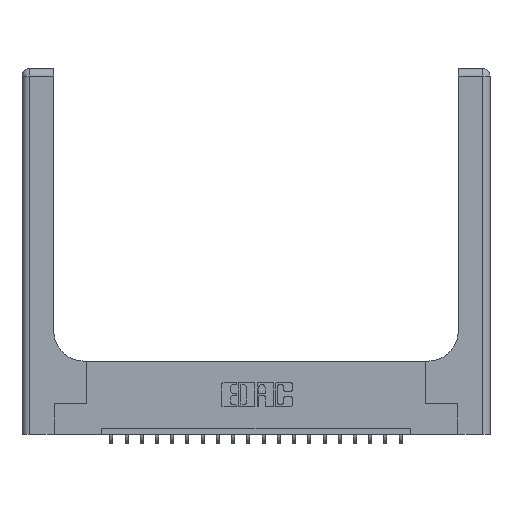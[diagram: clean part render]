
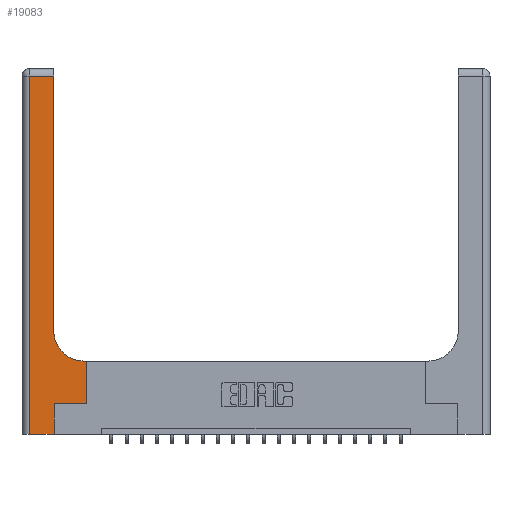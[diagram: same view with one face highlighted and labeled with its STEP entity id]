
A CAD part, top view. The second image highlights one B-rep face of the part: STEP entity #19083.
In plain terms, the highlighted planar face has unit normal (0, 0, 1).
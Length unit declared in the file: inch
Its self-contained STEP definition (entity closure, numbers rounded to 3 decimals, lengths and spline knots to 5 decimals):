
#293 = DIRECTION ( 'NONE',  ( 1., 0., 0. ) ) ;
#613 = DIRECTION ( 'NONE',  ( 0., 0., -1. ) ) ;
#1088 = VECTOR ( 'NONE', #14825, 39.37008 ) ;
#1104 = CARTESIAN_POINT ( 'NONE',  ( 0., 2.94, 0.37 ) ) ;
#1169 = ORIENTED_EDGE ( 'NONE', *, *, #7126, .T. ) ;
#1303 = VECTOR ( 'NONE', #6247, 39.37008 ) ;
#1861 = VERTEX_POINT ( 'NONE', #7684 ) ;
#1907 = CARTESIAN_POINT ( 'NONE',  ( 0.51, 0.85, 0.37 ) ) ;
#2509 = DIRECTION ( 'NONE',  ( -1., 0., 0. ) ) ;
#2930 = ORIENTED_EDGE ( 'NONE', *, *, #20727, .T. ) ;
#3854 = ORIENTED_EDGE ( 'NONE', *, *, #9664, .T. ) ;
#4037 = EDGE_CURVE ( 'NONE', #7189, #21075, #8366, .T. ) ;
#4624 = FACE_OUTER_BOUND ( 'NONE', #9613, .T. ) ;
#4665 = EDGE_CURVE ( 'NONE', #15276, #17112, #15567, .T. ) ;
#4895 = VERTEX_POINT ( 'NONE', #20072 ) ;
#6247 = DIRECTION ( 'NONE',  ( 0., -1., 0. ) ) ;
#6310 = CARTESIAN_POINT ( 'NONE',  ( 0.26, 3., 0.37 ) ) ;
#6574 = CARTESIAN_POINT ( 'NONE',  ( 0.26, 0.6, 0.37 ) ) ;
#6630 = CARTESIAN_POINT ( 'NONE',  ( 0.528, 0.25, 0.37 ) ) ;
#6782 = LINE ( 'NONE', #6574, #1088 ) ;
#7012 = ORIENTED_EDGE ( 'NONE', *, *, #15500, .T. ) ;
#7126 = EDGE_CURVE ( 'NONE', #17112, #9263, #20725, .T. ) ;
#7189 = VERTEX_POINT ( 'NONE', #19460 ) ;
#7630 = PLANE ( 'NONE',  #12415 ) ;
#7684 = CARTESIAN_POINT ( 'NONE',  ( 0.26, 0.85, 0.37 ) ) ;
#7922 = VECTOR ( 'NONE', #16930, 39.37008 ) ;
#7959 = VERTEX_POINT ( 'NONE', #14280 ) ;
#8366 = LINE ( 'NONE', #18451, #14197 ) ;
#8649 = CARTESIAN_POINT ( 'NONE',  ( 0.265, 0., 0.37 ) ) ;
#8744 = ORIENTED_EDGE ( 'NONE', *, *, #4037, .T. ) ;
#8818 = EDGE_CURVE ( 'NONE', #21075, #4895, #17923, .T. ) ;
#9263 = VERTEX_POINT ( 'NONE', #14306 ) ;
#9374 = EDGE_CURVE ( 'NONE', #7959, #1861, #20838, .T. ) ;
#9612 = CARTESIAN_POINT ( 'NONE',  ( 0.06, 2.94, 0.37 ) ) ;
#9613 = EDGE_LOOP ( 'NONE', ( #2930, #11601, #1169, #10731, #7012, #8744, #12148, #3854, #19060 ) ) ;
#9664 = EDGE_CURVE ( 'NONE', #4895, #7959, #6782, .T. ) ;
#10173 = DIRECTION ( 'NONE',  ( 1., 0., 0. ) ) ;
#10459 = LINE ( 'NONE', #8649, #7922 ) ;
#10731 = ORIENTED_EDGE ( 'NONE', *, *, #20761, .T. ) ;
#11212 = CARTESIAN_POINT ( 'NONE',  ( 0.528, 0.25, 0.37 ) ) ;
#11262 = CARTESIAN_POINT ( 'NONE',  ( 0., 3., 0.37 ) ) ;
#11339 = AXIS2_PLACEMENT_3D ( 'NONE', #1907, #613, #293 ) ;
#11601 = ORIENTED_EDGE ( 'NONE', *, *, #4665, .T. ) ;
#11737 = VECTOR ( 'NONE', #12838, 39.37008 ) ;
#12148 = ORIENTED_EDGE ( 'NONE', *, *, #8818, .T. ) ;
#12415 = AXIS2_PLACEMENT_3D ( 'NONE', #11262, #20925, #14150 ) ;
#12625 = LINE ( 'NONE', #6310, #11737 ) ;
#12838 = DIRECTION ( 'NONE',  ( 0., 1., 0. ) ) ;
#13162 = DIRECTION ( 'NONE',  ( 0., 1., 0. ) ) ;
#14006 = VECTOR ( 'NONE', #13162, 39.37008 ) ;
#14150 = DIRECTION ( 'NONE',  ( -1., 0., 0. ) ) ;
#14197 = VECTOR ( 'NONE', #10173, 39.37008 ) ;
#14280 = CARTESIAN_POINT ( 'NONE',  ( 0.51, 0.6, 0.37 ) ) ;
#14306 = CARTESIAN_POINT ( 'NONE',  ( 0.06, 0., 0.37 ) ) ;
#14825 = DIRECTION ( 'NONE',  ( -1., 0., 0. ) ) ;
#15276 = VERTEX_POINT ( 'NONE', #17991 ) ;
#15500 = EDGE_CURVE ( 'NONE', #15914, #7189, #10459, .T. ) ;
#15567 = LINE ( 'NONE', #1104, #18614 ) ;
#15914 = VERTEX_POINT ( 'NONE', #18074 ) ;
#16930 = DIRECTION ( 'NONE',  ( 0., 1., 0. ) ) ;
#17112 = VERTEX_POINT ( 'NONE', #9612 ) ;
#17923 = LINE ( 'NONE', #6630, #14006 ) ;
#17991 = CARTESIAN_POINT ( 'NONE',  ( 0.26, 2.94, 0.37 ) ) ;
#18074 = CARTESIAN_POINT ( 'NONE',  ( 0.265, 0., 0.37 ) ) ;
#18138 = CARTESIAN_POINT ( 'NONE',  ( 0., 0., 0.37 ) ) ;
#18238 = DIRECTION ( 'NONE',  ( 1., 0., 0. ) ) ;
#18451 = CARTESIAN_POINT ( 'NONE',  ( 0.265, 0.25, 0.37 ) ) ;
#18614 = VECTOR ( 'NONE', #2509, 39.37008 ) ;
#19060 = ORIENTED_EDGE ( 'NONE', *, *, #9374, .T. ) ;
#19083 = ADVANCED_FACE ( 'NONE', ( #4624 ), #7630, .F. ) ;
#19460 = CARTESIAN_POINT ( 'NONE',  ( 0.265, 0.25, 0.37 ) ) ;
#19522 = VECTOR ( 'NONE', #18238, 39.37008 ) ;
#19721 = LINE ( 'NONE', #18138, #19522 ) ;
#20072 = CARTESIAN_POINT ( 'NONE',  ( 0.528, 0.6, 0.37 ) ) ;
#20725 = LINE ( 'NONE', #20944, #1303 ) ;
#20727 = EDGE_CURVE ( 'NONE', #1861, #15276, #12625, .T. ) ;
#20761 = EDGE_CURVE ( 'NONE', #9263, #15914, #19721, .T. ) ;
#20838 = CIRCLE ( 'NONE', #11339, 0.25 ) ;
#20925 = DIRECTION ( 'NONE',  ( 0., 0., -1. ) ) ;
#20944 = CARTESIAN_POINT ( 'NONE',  ( 0.06, 3., 0.37 ) ) ;
#21075 = VERTEX_POINT ( 'NONE', #11212 ) ;
